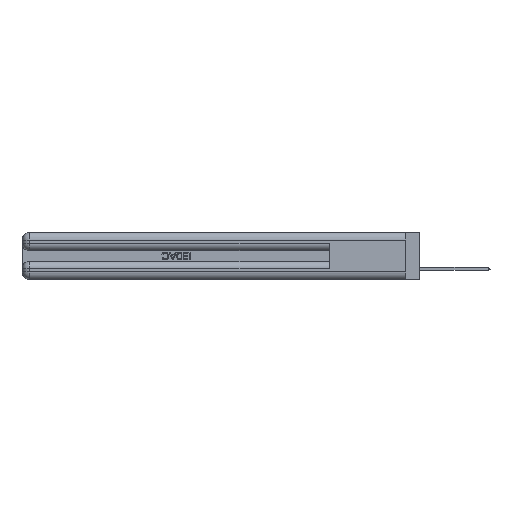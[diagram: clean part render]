
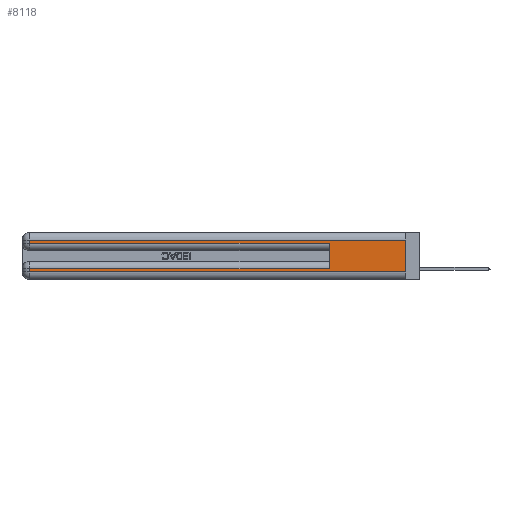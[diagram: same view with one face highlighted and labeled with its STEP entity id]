
A CAD part, left-side view. The second image highlights one B-rep face of the part: STEP entity #8118.
In plain terms, the highlighted planar face has unit normal (-1, 0, 0).
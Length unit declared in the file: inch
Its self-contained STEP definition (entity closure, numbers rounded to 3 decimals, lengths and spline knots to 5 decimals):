
#24 = CARTESIAN_POINT ( 'NONE',  ( 0., 2.94, 0.085 ) ) ;
#1523 = EDGE_CURVE ( 'NONE', #38134, #23130, #2375, .T. ) ;
#2375 = LINE ( 'NONE', #2842, #5412 ) ;
#2513 = DIRECTION ( 'NONE',  ( 0., -1., 0. ) ) ;
#2842 = CARTESIAN_POINT ( 'NONE',  ( 0., 2.94, 0.37 ) ) ;
#2875 = ORIENTED_EDGE ( 'NONE', *, *, #35269, .F. ) ;
#3107 = DIRECTION ( 'NONE',  ( 0., 1., 0. ) ) ;
#3380 = CARTESIAN_POINT ( 'NONE',  ( 0., 0., 0.37 ) ) ;
#4824 = ORIENTED_EDGE ( 'NONE', *, *, #1523, .T. ) ;
#5412 = VECTOR ( 'NONE', #30329, 39.37008 ) ;
#5869 = ORIENTED_EDGE ( 'NONE', *, *, #6091, .T. ) ;
#6091 = EDGE_CURVE ( 'NONE', #18134, #11733, #20725, .T. ) ;
#6274 = LINE ( 'NONE', #26474, #25778 ) ;
#6794 = VECTOR ( 'NONE', #33011, 39.37008 ) ;
#7994 = LINE ( 'NONE', #47321, #6794 ) ;
#8118 = ADVANCED_FACE ( 'NONE', ( #16411 ), #49733, .F. ) ;
#9484 = CARTESIAN_POINT ( 'NONE',  ( 0., 2.94, 0.37 ) ) ;
#9653 = ORIENTED_EDGE ( 'NONE', *, *, #21124, .F. ) ;
#11733 = VERTEX_POINT ( 'NONE', #25292 ) ;
#13160 = CARTESIAN_POINT ( 'NONE',  ( 0., 2.94, 0.06 ) ) ;
#16004 = LINE ( 'NONE', #21965, #25851 ) ;
#16404 = VECTOR ( 'NONE', #36795, 39.37008 ) ;
#16411 = FACE_OUTER_BOUND ( 'NONE', #17589, .T. ) ;
#17589 = EDGE_LOOP ( 'NONE', ( #2875, #33629, #5869, #45837, #9653, #49271, #4824, #27896 ) ) ;
#18134 = VERTEX_POINT ( 'NONE', #40561 ) ;
#19574 = CARTESIAN_POINT ( 'NONE',  ( 0., 0., 0.31 ) ) ;
#20725 = LINE ( 'NONE', #9484, #16404 ) ;
#21124 = EDGE_CURVE ( 'NONE', #33458, #37991, #16004, .T. ) ;
#21965 = CARTESIAN_POINT ( 'NONE',  ( 0., 0.6, 0.145 ) ) ;
#22588 = DIRECTION ( 'NONE',  ( 0., 0., -1. ) ) ;
#23130 = VERTEX_POINT ( 'NONE', #13160 ) ;
#24391 = AXIS2_PLACEMENT_3D ( 'NONE', #3380, #24422, #22588 ) ;
#24422 = DIRECTION ( 'NONE',  ( 1., 0., 0. ) ) ;
#24649 = VERTEX_POINT ( 'NONE', #40708 ) ;
#25292 = CARTESIAN_POINT ( 'NONE',  ( 0., 2.94, 0.285 ) ) ;
#25778 = VECTOR ( 'NONE', #3107, 39.37008 ) ;
#25851 = VECTOR ( 'NONE', #39997, 39.37008 ) ;
#26474 = CARTESIAN_POINT ( 'NONE',  ( 0., 0., 0.085 ) ) ;
#27253 = VERTEX_POINT ( 'NONE', #19574 ) ;
#27896 = ORIENTED_EDGE ( 'NONE', *, *, #36136, .T. ) ;
#28003 = LINE ( 'NONE', #31766, #30533 ) ;
#29661 = CARTESIAN_POINT ( 'NONE',  ( 0., 0., 0.06 ) ) ;
#30329 = DIRECTION ( 'NONE',  ( 0., 0., -1. ) ) ;
#30533 = VECTOR ( 'NONE', #43857, 39.37008 ) ;
#31278 = EDGE_CURVE ( 'NONE', #27253, #18134, #37234, .T. ) ;
#31725 = VECTOR ( 'NONE', #48857, 39.37008 ) ;
#31746 = EDGE_CURVE ( 'NONE', #11733, #37991, #7994, .T. ) ;
#31766 = CARTESIAN_POINT ( 'NONE',  ( 0., 0., 0.37 ) ) ;
#33011 = DIRECTION ( 'NONE',  ( 0., -1., 0. ) ) ;
#33458 = VERTEX_POINT ( 'NONE', #43390 ) ;
#33629 = ORIENTED_EDGE ( 'NONE', *, *, #31278, .T. ) ;
#34673 = LINE ( 'NONE', #29661, #47438 ) ;
#35269 = EDGE_CURVE ( 'NONE', #27253, #24649, #28003, .T. ) ;
#36136 = EDGE_CURVE ( 'NONE', #23130, #24649, #34673, .T. ) ;
#36795 = DIRECTION ( 'NONE',  ( 0., 0., -1. ) ) ;
#37234 = LINE ( 'NONE', #49033, #31725 ) ;
#37991 = VERTEX_POINT ( 'NONE', #46139 ) ;
#38134 = VERTEX_POINT ( 'NONE', #24 ) ;
#39997 = DIRECTION ( 'NONE',  ( 0., 0., 1. ) ) ;
#40561 = CARTESIAN_POINT ( 'NONE',  ( 0., 2.94, 0.31 ) ) ;
#40708 = CARTESIAN_POINT ( 'NONE',  ( 0., 0., 0.06 ) ) ;
#43070 = EDGE_CURVE ( 'NONE', #33458, #38134, #6274, .T. ) ;
#43390 = CARTESIAN_POINT ( 'NONE',  ( 0., 0.6, 0.085 ) ) ;
#43857 = DIRECTION ( 'NONE',  ( 0., 0., -1. ) ) ;
#45837 = ORIENTED_EDGE ( 'NONE', *, *, #31746, .T. ) ;
#46139 = CARTESIAN_POINT ( 'NONE',  ( 0., 0.6, 0.285 ) ) ;
#47321 = CARTESIAN_POINT ( 'NONE',  ( 0., 0., 0.285 ) ) ;
#47438 = VECTOR ( 'NONE', #2513, 39.37008 ) ;
#48857 = DIRECTION ( 'NONE',  ( 0., 1., 0. ) ) ;
#49033 = CARTESIAN_POINT ( 'NONE',  ( 0., 0., 0.31 ) ) ;
#49271 = ORIENTED_EDGE ( 'NONE', *, *, #43070, .T. ) ;
#49733 = PLANE ( 'NONE',  #24391 ) ;
